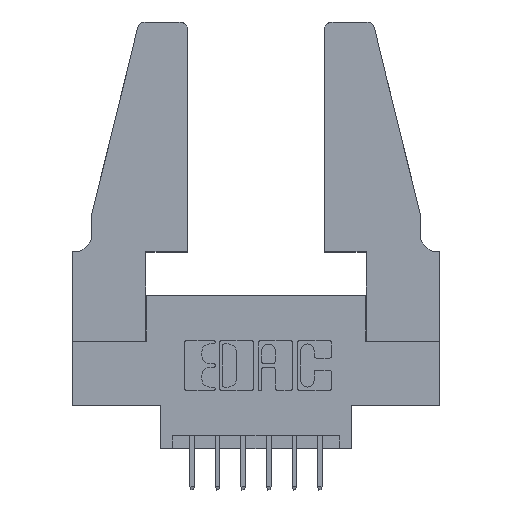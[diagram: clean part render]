
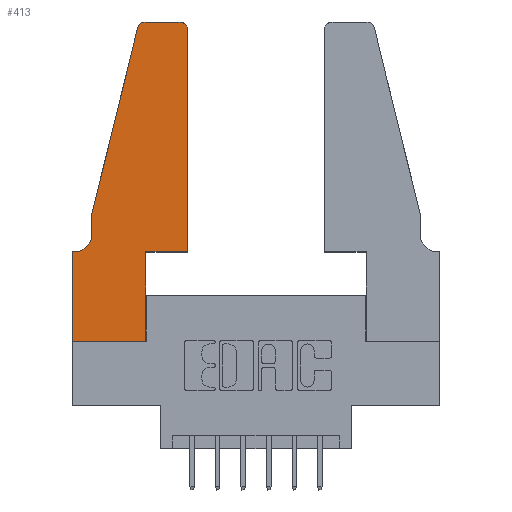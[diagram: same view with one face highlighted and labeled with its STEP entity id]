
A CAD part, top view. The second image highlights one B-rep face of the part: STEP entity #413.
In plain terms, the highlighted planar face has unit normal (0, 0, 1).
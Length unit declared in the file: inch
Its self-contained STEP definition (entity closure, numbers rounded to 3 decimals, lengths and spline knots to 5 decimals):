
#37 = CARTESIAN_POINT ( 'NONE',  ( 0.284, 1.25, 0.37 ) ) ;
#135 = ORIENTED_EDGE ( 'NONE', *, *, #1275, .T. ) ;
#163 = VERTEX_POINT ( 'NONE', #9241 ) ;
#413 = ADVANCED_FACE ( 'NONE', ( #5030 ), #10948, .T. ) ;
#431 = VERTEX_POINT ( 'NONE', #9755 ) ;
#433 = ORIENTED_EDGE ( 'NONE', *, *, #7775, .T. ) ;
#494 = LINE ( 'NONE', #10673, #7652 ) ;
#608 = CARTESIAN_POINT ( 'NONE',  ( 0.0755, 0.42, 0.37 ) ) ;
#685 = EDGE_CURVE ( 'NONE', #1097, #9434, #6990, .T. ) ;
#837 = CARTESIAN_POINT ( 'NONE',  ( 0.25487, 1.22718, 0.37 ) ) ;
#1058 = ORIENTED_EDGE ( 'NONE', *, *, #5397, .T. ) ;
#1097 = VERTEX_POINT ( 'NONE', #10457 ) ;
#1163 = DIRECTION ( 'NONE',  ( 1., 0., 0. ) ) ;
#1188 = EDGE_CURVE ( 'NONE', #7649, #5297, #4887, .T. ) ;
#1275 = EDGE_CURVE ( 'NONE', #5297, #431, #2357, .T. ) ;
#1446 = VECTOR ( 'NONE', #2752, 39.37008 ) ;
#1491 = CARTESIAN_POINT ( 'NONE',  ( 0.2605, 1.25, 0.37 ) ) ;
#1909 = DIRECTION ( 'NONE',  ( 1., 0., 0. ) ) ;
#1949 = DIRECTION ( 'NONE',  ( 0., 0., 1. ) ) ;
#1969 = DIRECTION ( 'NONE',  ( 0., 1., 0. ) ) ;
#2056 = CARTESIAN_POINT ( 'NONE',  ( 0.284, 1.22, 0.37 ) ) ;
#2357 = LINE ( 'NONE', #6903, #1446 ) ;
#2468 = LINE ( 'NONE', #3171, #7086 ) ;
#2728 = ORIENTED_EDGE ( 'NONE', *, *, #10548, .T. ) ;
#2748 = DIRECTION ( 'NONE',  ( 1., 0., 0. ) ) ;
#2752 = DIRECTION ( 'NONE',  ( -0.239, -0.971, 0. ) ) ;
#2925 = DIRECTION ( 'NONE',  ( 0., 1., 0. ) ) ;
#3111 = CARTESIAN_POINT ( 'NONE',  ( 0., 0.35, 0.37 ) ) ;
#3171 = CARTESIAN_POINT ( 'NONE',  ( 0., 0., 0.37 ) ) ;
#3335 = ORIENTED_EDGE ( 'NONE', *, *, #7993, .T. ) ;
#3500 = DIRECTION ( 'NONE',  ( 0., -1., 0. ) ) ;
#3517 = AXIS2_PLACEMENT_3D ( 'NONE', #2056, #1949, #1909 ) ;
#3577 = CARTESIAN_POINT ( 'NONE',  ( 0.2865, 0., 0.37 ) ) ;
#3611 = EDGE_CURVE ( 'NONE', #7720, #11801, #2468, .T. ) ;
#3617 = ORIENTED_EDGE ( 'NONE', *, *, #685, .T. ) ;
#3619 = DIRECTION ( 'NONE',  ( 1., 0., 0. ) ) ;
#3707 = CARTESIAN_POINT ( 'NONE',  ( 0.4505, 0.35, 0.37 ) ) ;
#3725 = VERTEX_POINT ( 'NONE', #4307 ) ;
#4080 = LINE ( 'NONE', #10209, #6485 ) ;
#4215 = CIRCLE ( 'NONE', #5086, 0.07 ) ;
#4307 = CARTESIAN_POINT ( 'NONE',  ( 0.4505, 0.35, 0.37 ) ) ;
#4887 = CIRCLE ( 'NONE', #3517, 0.03 ) ;
#4890 = LINE ( 'NONE', #7316, #11763 ) ;
#4932 = ORIENTED_EDGE ( 'NONE', *, *, #11129, .T. ) ;
#5026 = VECTOR ( 'NONE', #5956, 39.37008 ) ;
#5029 = DIRECTION ( 'NONE',  ( 0., 0., 1. ) ) ;
#5030 = FACE_OUTER_BOUND ( 'NONE', #10322, .T. ) ;
#5086 = AXIS2_PLACEMENT_3D ( 'NONE', #10517, #5145, #11422 ) ;
#5145 = DIRECTION ( 'NONE',  ( 0., 0., -1. ) ) ;
#5157 = CARTESIAN_POINT ( 'NONE',  ( 0.4205, 1.22, 0.37 ) ) ;
#5297 = VERTEX_POINT ( 'NONE', #837 ) ;
#5397 = EDGE_CURVE ( 'NONE', #3725, #1097, #4080, .T. ) ;
#5492 = ORIENTED_EDGE ( 'NONE', *, *, #3611, .T. ) ;
#5614 = EDGE_CURVE ( 'NONE', #8475, #7980, #4215, .T. ) ;
#5778 = ORIENTED_EDGE ( 'NONE', *, *, #10802, .T. ) ;
#5956 = DIRECTION ( 'NONE',  ( -1., 0., 0. ) ) ;
#5959 = VECTOR ( 'NONE', #9747, 39.37008 ) ;
#6485 = VECTOR ( 'NONE', #2925, 39.37008 ) ;
#6751 = VERTEX_POINT ( 'NONE', #3577 ) ;
#6873 = EDGE_CURVE ( 'NONE', #163, #3725, #7704, .T. ) ;
#6903 = CARTESIAN_POINT ( 'NONE',  ( 0.0755, 0.5, 0.37 ) ) ;
#6990 = CIRCLE ( 'NONE', #7013, 0.03 ) ;
#7013 = AXIS2_PLACEMENT_3D ( 'NONE', #5157, #5029, #3619 ) ;
#7086 = VECTOR ( 'NONE', #7729, 39.37008 ) ;
#7227 = AXIS2_PLACEMENT_3D ( 'NONE', #11043, #10923, #1163 ) ;
#7306 = ORIENTED_EDGE ( 'NONE', *, *, #1188, .T. ) ;
#7316 = CARTESIAN_POINT ( 'NONE',  ( 0., 0., 0.37 ) ) ;
#7495 = CARTESIAN_POINT ( 'NONE',  ( 0.2865, 0.35, 0.37 ) ) ;
#7649 = VERTEX_POINT ( 'NONE', #37 ) ;
#7652 = VECTOR ( 'NONE', #3500, 39.37008 ) ;
#7704 = LINE ( 'NONE', #3707, #10095 ) ;
#7720 = VERTEX_POINT ( 'NONE', #3111 ) ;
#7729 = DIRECTION ( 'NONE',  ( 0., -1., 0. ) ) ;
#7775 = EDGE_CURVE ( 'NONE', #7980, #7720, #9484, .T. ) ;
#7980 = VERTEX_POINT ( 'NONE', #10895 ) ;
#7993 = EDGE_CURVE ( 'NONE', #11801, #6751, #4890, .T. ) ;
#8205 = DIRECTION ( 'NONE',  ( 1., 0., 0. ) ) ;
#8319 = LINE ( 'NONE', #1491, #5959 ) ;
#8330 = CARTESIAN_POINT ( 'NONE',  ( 0.4205, 1.25, 0.37 ) ) ;
#8475 = VERTEX_POINT ( 'NONE', #608 ) ;
#9048 = CARTESIAN_POINT ( 'NONE',  ( 0., 0., 0.37 ) ) ;
#9241 = CARTESIAN_POINT ( 'NONE',  ( 0.2865, 0.35, 0.37 ) ) ;
#9301 = LINE ( 'NONE', #7495, #11715 ) ;
#9434 = VERTEX_POINT ( 'NONE', #8330 ) ;
#9484 = LINE ( 'NONE', #11336, #5026 ) ;
#9747 = DIRECTION ( 'NONE',  ( -1., 0., 0. ) ) ;
#9755 = CARTESIAN_POINT ( 'NONE',  ( 0.0755, 0.5, 0.37 ) ) ;
#9963 = ORIENTED_EDGE ( 'NONE', *, *, #5614, .T. ) ;
#10095 = VECTOR ( 'NONE', #2748, 39.37008 ) ;
#10209 = CARTESIAN_POINT ( 'NONE',  ( 0.4505, 0.35, 0.37 ) ) ;
#10322 = EDGE_LOOP ( 'NONE', ( #4932, #7306, #135, #2728, #9963, #433, #5492, #3335, #5778, #10533, #1058, #3617 ) ) ;
#10457 = CARTESIAN_POINT ( 'NONE',  ( 0.4505, 1.22, 0.37 ) ) ;
#10517 = CARTESIAN_POINT ( 'NONE',  ( 0.0055, 0.42, 0.37 ) ) ;
#10533 = ORIENTED_EDGE ( 'NONE', *, *, #6873, .T. ) ;
#10548 = EDGE_CURVE ( 'NONE', #431, #8475, #494, .T. ) ;
#10673 = CARTESIAN_POINT ( 'NONE',  ( 0.0755, 0.5, 0.37 ) ) ;
#10802 = EDGE_CURVE ( 'NONE', #6751, #163, #9301, .T. ) ;
#10895 = CARTESIAN_POINT ( 'NONE',  ( 0.0055, 0.35, 0.37 ) ) ;
#10923 = DIRECTION ( 'NONE',  ( 0., 0., 1. ) ) ;
#10948 = PLANE ( 'NONE',  #7227 ) ;
#11043 = CARTESIAN_POINT ( 'NONE',  ( 0., 0.35, 0.37 ) ) ;
#11129 = EDGE_CURVE ( 'NONE', #9434, #7649, #8319, .T. ) ;
#11336 = CARTESIAN_POINT ( 'NONE',  ( 0.0755, 0.35, 0.37 ) ) ;
#11422 = DIRECTION ( 'NONE',  ( -1., 0., 0. ) ) ;
#11715 = VECTOR ( 'NONE', #1969, 39.37008 ) ;
#11763 = VECTOR ( 'NONE', #8205, 39.37008 ) ;
#11801 = VERTEX_POINT ( 'NONE', #9048 ) ;
